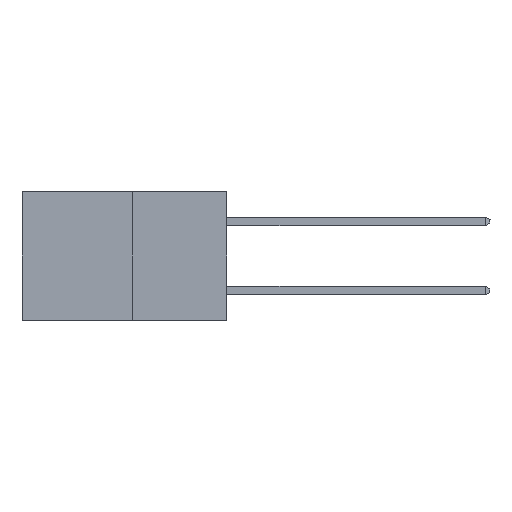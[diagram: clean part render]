
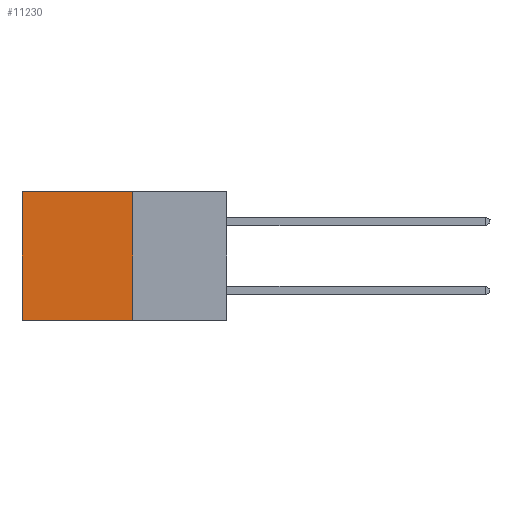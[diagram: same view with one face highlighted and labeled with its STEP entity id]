
A CAD part, left-side view. The second image highlights one B-rep face of the part: STEP entity #11230.
In plain terms, the highlighted planar face has unit normal (-1, 0, 0).
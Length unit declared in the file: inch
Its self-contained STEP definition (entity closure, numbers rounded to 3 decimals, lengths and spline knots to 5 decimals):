
#15 = VERTEX_POINT ( 'NONE', #840 ) ;
#840 = CARTESIAN_POINT ( 'NONE',  ( 0.277, 0.27, 0. ) ) ;
#918 = ORIENTED_EDGE ( 'NONE', *, *, #13427, .F. ) ;
#969 = ORIENTED_EDGE ( 'NONE', *, *, #11948, .T. ) ;
#1603 = DIRECTION ( 'NONE',  ( 1., 0., 0. ) ) ;
#1850 = VECTOR ( 'NONE', #8950, 39.37008 ) ;
#2106 = ORIENTED_EDGE ( 'NONE', *, *, #6884, .T. ) ;
#2244 = VERTEX_POINT ( 'NONE', #6862 ) ;
#2471 = VECTOR ( 'NONE', #13675, 39.37008 ) ;
#2752 = AXIS2_PLACEMENT_3D ( 'NONE', #7233, #1603, #9491 ) ;
#2792 = EDGE_CURVE ( 'NONE', #2244, #9717, #4605, .T. ) ;
#2804 = VECTOR ( 'NONE', #12834, 39.37008 ) ;
#3203 = CARTESIAN_POINT ( 'NONE',  ( 0.277, 0.27, -0.37 ) ) ;
#3975 = VERTEX_POINT ( 'NONE', #5515 ) ;
#4605 = LINE ( 'NONE', #3203, #10220 ) ;
#4639 = DIRECTION ( 'NONE',  ( 0., 1., 0. ) ) ;
#4868 = CARTESIAN_POINT ( 'NONE',  ( 0.277, 0.59, -0.37 ) ) ;
#5199 = LINE ( 'NONE', #9800, #1850 ) ;
#5515 = CARTESIAN_POINT ( 'NONE',  ( 0.277, 0.59, 0. ) ) ;
#5796 = LINE ( 'NONE', #12877, #2804 ) ;
#6774 = EDGE_LOOP ( 'NONE', ( #969, #8662, #918, #2106 ) ) ;
#6862 = CARTESIAN_POINT ( 'NONE',  ( 0.277, 0.27, -0.37 ) ) ;
#6884 = EDGE_CURVE ( 'NONE', #15, #3975, #5199, .T. ) ;
#7233 = CARTESIAN_POINT ( 'NONE',  ( 0.277, 0.27, -0.37 ) ) ;
#8397 = PLANE ( 'NONE',  #2752 ) ;
#8662 = ORIENTED_EDGE ( 'NONE', *, *, #2792, .F. ) ;
#8950 = DIRECTION ( 'NONE',  ( 0., 1., 0. ) ) ;
#9076 = FACE_OUTER_BOUND ( 'NONE', #6774, .T. ) ;
#9491 = DIRECTION ( 'NONE',  ( 0., 0., -1. ) ) ;
#9717 = VERTEX_POINT ( 'NONE', #9990 ) ;
#9800 = CARTESIAN_POINT ( 'NONE',  ( 0.277, 0.27, 0. ) ) ;
#9990 = CARTESIAN_POINT ( 'NONE',  ( 0.277, 0.59, -0.37 ) ) ;
#10220 = VECTOR ( 'NONE', #4639, 39.37008 ) ;
#11230 = ADVANCED_FACE ( 'NONE', ( #9076 ), #8397, .F. ) ;
#11429 = LINE ( 'NONE', #4868, #2471 ) ;
#11948 = EDGE_CURVE ( 'NONE', #3975, #9717, #11429, .T. ) ;
#12834 = DIRECTION ( 'NONE',  ( 0., 0., -1. ) ) ;
#12877 = CARTESIAN_POINT ( 'NONE',  ( 0.277, 0.27, -0.37 ) ) ;
#13427 = EDGE_CURVE ( 'NONE', #15, #2244, #5796, .T. ) ;
#13675 = DIRECTION ( 'NONE',  ( 0., 0., -1. ) ) ;
